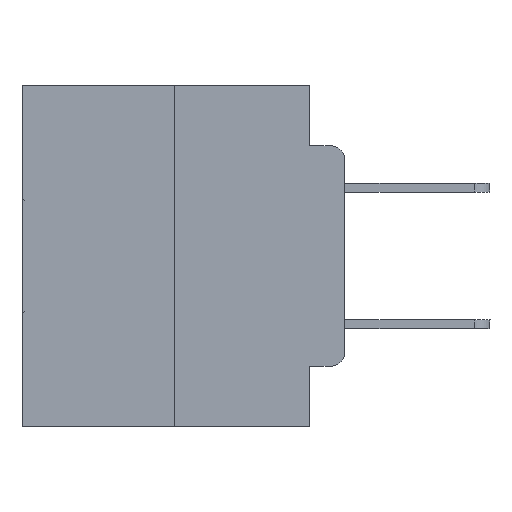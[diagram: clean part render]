
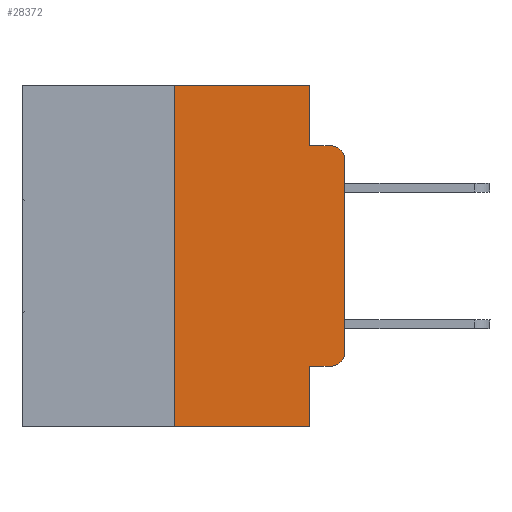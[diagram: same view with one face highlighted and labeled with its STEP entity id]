
A CAD part, left-side view. The second image highlights one B-rep face of the part: STEP entity #28372.
In plain terms, the highlighted planar face has unit normal (-1, 0, 0).
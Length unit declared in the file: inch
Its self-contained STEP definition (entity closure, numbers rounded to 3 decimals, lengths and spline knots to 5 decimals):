
#468 = CARTESIAN_POINT ( 'NONE',  ( 0., 0.051, -0.5 ) ) ;
#787 = DIRECTION ( 'NONE',  ( 1., 0., 0. ) ) ;
#1139 = VECTOR ( 'NONE', #12857, 39.37008 ) ;
#1265 = ORIENTED_EDGE ( 'NONE', *, *, #15100, .F. ) ;
#1633 = CARTESIAN_POINT ( 'NONE',  ( 0., 0.051, -0.0885 ) ) ;
#2625 = DIRECTION ( 'NONE',  ( 0., 0., -1. ) ) ;
#2708 = DIRECTION ( 'NONE',  ( 0., -1., 0. ) ) ;
#2713 = VECTOR ( 'NONE', #7961, 39.37008 ) ;
#2823 = DIRECTION ( 'NONE',  ( 0., -1., 0. ) ) ;
#2916 = AXIS2_PLACEMENT_3D ( 'NONE', #28084, #3341, #10040 ) ;
#3341 = DIRECTION ( 'NONE',  ( -1., 0., 0. ) ) ;
#3675 = DIRECTION ( 'NONE',  ( 0., 0., -1. ) ) ;
#3741 = CARTESIAN_POINT ( 'NONE',  ( 0., 0.25, 0. ) ) ;
#3855 = VECTOR ( 'NONE', #2708, 39.37008 ) ;
#3973 = CARTESIAN_POINT ( 'NONE',  ( 0., 0., 0. ) ) ;
#4028 = EDGE_CURVE ( 'NONE', #7011, #19054, #7612, .T. ) ;
#4099 = VERTEX_POINT ( 'NONE', #1633 ) ;
#4632 = ORIENTED_EDGE ( 'NONE', *, *, #24518, .F. ) ;
#4647 = CARTESIAN_POINT ( 'NONE',  ( 0., 0.02, -0.0885 ) ) ;
#4889 = CARTESIAN_POINT ( 'NONE',  ( 0., 0.473, 0. ) ) ;
#5433 = EDGE_CURVE ( 'NONE', #12659, #21714, #24053, .T. ) ;
#5508 = LINE ( 'NONE', #5807, #8513 ) ;
#5686 = VERTEX_POINT ( 'NONE', #7299 ) ;
#5807 = CARTESIAN_POINT ( 'NONE',  ( 0., 0.051, 0. ) ) ;
#5992 = VERTEX_POINT ( 'NONE', #4647 ) ;
#6786 = LINE ( 'NONE', #20699, #3855 ) ;
#7011 = VERTEX_POINT ( 'NONE', #27759 ) ;
#7183 = AXIS2_PLACEMENT_3D ( 'NONE', #4889, #787, #3675 ) ;
#7297 = EDGE_CURVE ( 'NONE', #28199, #5686, #6786, .T. ) ;
#7299 = CARTESIAN_POINT ( 'NONE',  ( 0., 0.051, 0. ) ) ;
#7456 = CARTESIAN_POINT ( 'NONE',  ( 0., 0.051, -0.4115 ) ) ;
#7608 = DIRECTION ( 'NONE',  ( 0., 0., -1. ) ) ;
#7612 = LINE ( 'NONE', #16690, #20331 ) ;
#7642 = VERTEX_POINT ( 'NONE', #7456 ) ;
#7725 = EDGE_CURVE ( 'NONE', #21714, #5992, #9422, .T. ) ;
#7947 = CARTESIAN_POINT ( 'NONE',  ( 0., 0., -0.1085 ) ) ;
#7961 = DIRECTION ( 'NONE',  ( 0., -1., 0. ) ) ;
#8513 = VECTOR ( 'NONE', #12501, 39.37008 ) ;
#9422 = CIRCLE ( 'NONE', #25831, 0.02 ) ;
#10040 = DIRECTION ( 'NONE',  ( 0., 0., -1. ) ) ;
#11431 = EDGE_LOOP ( 'NONE', ( #20588, #19953, #25278, #4632, #18111, #27551, #18092, #1265, #21037, #21108 ) ) ;
#11568 = CARTESIAN_POINT ( 'NONE',  ( 0., 0.02, -0.4115 ) ) ;
#11632 = CARTESIAN_POINT ( 'NONE',  ( 0., 0.051, 0. ) ) ;
#12031 = CARTESIAN_POINT ( 'NONE',  ( 0., 0.25, 0. ) ) ;
#12501 = DIRECTION ( 'NONE',  ( 0., 0., -1. ) ) ;
#12659 = VERTEX_POINT ( 'NONE', #17929 ) ;
#12857 = DIRECTION ( 'NONE',  ( 0., 0., 1. ) ) ;
#13106 = VERTEX_POINT ( 'NONE', #11568 ) ;
#13168 = CARTESIAN_POINT ( 'NONE',  ( 0., 0.051, -0.0885 ) ) ;
#14375 = VECTOR ( 'NONE', #20719, 39.37008 ) ;
#14455 = CARTESIAN_POINT ( 'NONE',  ( 0., 0.02, -0.1085 ) ) ;
#15100 = EDGE_CURVE ( 'NONE', #7642, #19054, #20469, .T. ) ;
#15198 = VECTOR ( 'NONE', #2625, 39.37008 ) ;
#15659 = EDGE_CURVE ( 'NONE', #7011, #28199, #27589, .T. ) ;
#16690 = CARTESIAN_POINT ( 'NONE',  ( 0., 0.473, -0.5 ) ) ;
#17929 = CARTESIAN_POINT ( 'NONE',  ( 0., 0., -0.3915 ) ) ;
#18092 = ORIENTED_EDGE ( 'NONE', *, *, #4028, .T. ) ;
#18111 = ORIENTED_EDGE ( 'NONE', *, *, #7297, .F. ) ;
#18437 = EDGE_CURVE ( 'NONE', #7642, #13106, #19100, .T. ) ;
#19054 = VERTEX_POINT ( 'NONE', #468 ) ;
#19100 = LINE ( 'NONE', #28050, #2713 ) ;
#19505 = DIRECTION ( 'NONE',  ( 0., -1., 0. ) ) ;
#19953 = ORIENTED_EDGE ( 'NONE', *, *, #7725, .T. ) ;
#20331 = VECTOR ( 'NONE', #2823, 39.37008 ) ;
#20469 = LINE ( 'NONE', #11632, #15198 ) ;
#20588 = ORIENTED_EDGE ( 'NONE', *, *, #5433, .T. ) ;
#20699 = CARTESIAN_POINT ( 'NONE',  ( 0., 0.473, 0. ) ) ;
#20719 = DIRECTION ( 'NONE',  ( 0., 0., 1. ) ) ;
#20843 = FACE_OUTER_BOUND ( 'NONE', #11431, .T. ) ;
#21037 = ORIENTED_EDGE ( 'NONE', *, *, #18437, .T. ) ;
#21108 = ORIENTED_EDGE ( 'NONE', *, *, #24540, .T. ) ;
#21714 = VERTEX_POINT ( 'NONE', #7947 ) ;
#21716 = LINE ( 'NONE', #13168, #28760 ) ;
#24053 = LINE ( 'NONE', #3973, #1139 ) ;
#24518 = EDGE_CURVE ( 'NONE', #5686, #4099, #5508, .T. ) ;
#24540 = EDGE_CURVE ( 'NONE', #13106, #12659, #28166, .T. ) ;
#25278 = ORIENTED_EDGE ( 'NONE', *, *, #26771, .F. ) ;
#25831 = AXIS2_PLACEMENT_3D ( 'NONE', #14455, #27985, #7608 ) ;
#26771 = EDGE_CURVE ( 'NONE', #4099, #5992, #21716, .T. ) ;
#27431 = PLANE ( 'NONE',  #7183 ) ;
#27551 = ORIENTED_EDGE ( 'NONE', *, *, #15659, .F. ) ;
#27589 = LINE ( 'NONE', #12031, #14375 ) ;
#27759 = CARTESIAN_POINT ( 'NONE',  ( 0., 0.25, -0.5 ) ) ;
#27985 = DIRECTION ( 'NONE',  ( -1., 0., 0. ) ) ;
#28050 = CARTESIAN_POINT ( 'NONE',  ( 0., 0.051, -0.4115 ) ) ;
#28084 = CARTESIAN_POINT ( 'NONE',  ( 0., 0.02, -0.3915 ) ) ;
#28166 = CIRCLE ( 'NONE', #2916, 0.02 ) ;
#28199 = VERTEX_POINT ( 'NONE', #3741 ) ;
#28372 = ADVANCED_FACE ( 'NONE', ( #20843 ), #27431, .F. ) ;
#28760 = VECTOR ( 'NONE', #19505, 39.37008 ) ;
